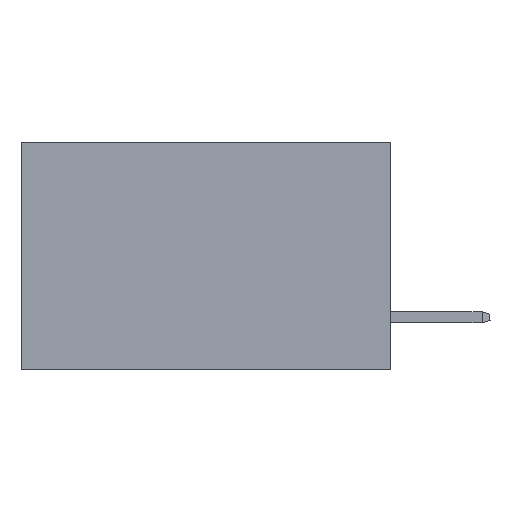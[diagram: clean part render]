
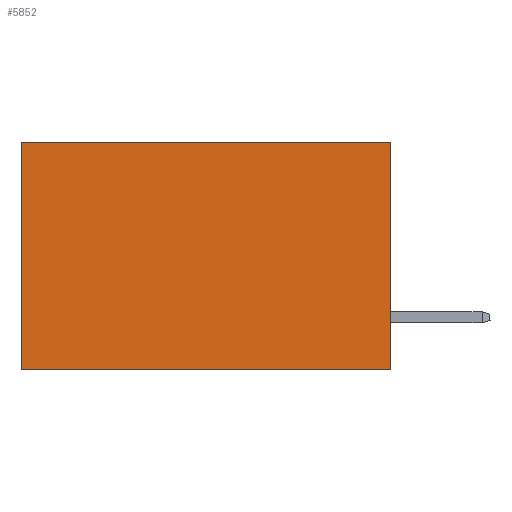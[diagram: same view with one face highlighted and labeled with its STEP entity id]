
A CAD part, left-side view. The second image highlights one B-rep face of the part: STEP entity #5852.
In plain terms, the highlighted planar face has unit normal (-1, 0, 0).
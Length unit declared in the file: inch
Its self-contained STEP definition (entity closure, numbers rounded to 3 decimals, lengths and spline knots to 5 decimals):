
#713 = VERTEX_POINT ( 'NONE', #25586 ) ;
#890 = VERTEX_POINT ( 'NONE', #19324 ) ;
#1612 = EDGE_CURVE ( 'NONE', #20987, #7884, #8159, .T. ) ;
#2070 = VECTOR ( 'NONE', #13593, 39.37008 ) ;
#2595 = EDGE_CURVE ( 'NONE', #890, #713, #14158, .T. ) ;
#3225 = EDGE_CURVE ( 'NONE', #890, #20987, #9853, .T. ) ;
#3799 = VECTOR ( 'NONE', #24616, 39.37008 ) ;
#4770 = EDGE_CURVE ( 'NONE', #713, #7884, #28774, .T. ) ;
#5852 = ADVANCED_FACE ( 'NONE', ( #21918 ), #17741, .F. ) ;
#6243 = DIRECTION ( 'NONE',  ( 1., 0., 0. ) ) ;
#7884 = VERTEX_POINT ( 'NONE', #21443 ) ;
#8159 = LINE ( 'NONE', #26647, #26771 ) ;
#8192 = ORIENTED_EDGE ( 'NONE', *, *, #3225, .T. ) ;
#8851 = CARTESIAN_POINT ( 'NONE',  ( 0.2875, 0., 0. ) ) ;
#8976 = DIRECTION ( 'NONE',  ( 0., 0., -1. ) ) ;
#9764 = DIRECTION ( 'NONE',  ( 0., 1., 0. ) ) ;
#9853 = LINE ( 'NONE', #8851, #3799 ) ;
#10595 = VECTOR ( 'NONE', #9764, 39.37008 ) ;
#11586 = ORIENTED_EDGE ( 'NONE', *, *, #4770, .F. ) ;
#12865 = DIRECTION ( 'NONE',  ( 0., 0., -1. ) ) ;
#13593 = DIRECTION ( 'NONE',  ( 0., 0., -1. ) ) ;
#13962 = CARTESIAN_POINT ( 'NONE',  ( 0.2875, 0., -0.37 ) ) ;
#14158 = LINE ( 'NONE', #17988, #2070 ) ;
#15620 = EDGE_LOOP ( 'NONE', ( #18037, #11586, #22037, #8192 ) ) ;
#17741 = PLANE ( 'NONE',  #24115 ) ;
#17988 = CARTESIAN_POINT ( 'NONE',  ( 0.2875, 0., 0. ) ) ;
#18037 = ORIENTED_EDGE ( 'NONE', *, *, #1612, .T. ) ;
#19324 = CARTESIAN_POINT ( 'NONE',  ( 0.2875, 0., 0. ) ) ;
#20016 = CARTESIAN_POINT ( 'NONE',  ( 0.2875, 0., 0. ) ) ;
#20987 = VERTEX_POINT ( 'NONE', #28680 ) ;
#21443 = CARTESIAN_POINT ( 'NONE',  ( 0.2875, 0.6, -0.37 ) ) ;
#21918 = FACE_OUTER_BOUND ( 'NONE', #15620, .T. ) ;
#22037 = ORIENTED_EDGE ( 'NONE', *, *, #2595, .F. ) ;
#24115 = AXIS2_PLACEMENT_3D ( 'NONE', #20016, #6243, #12865 ) ;
#24616 = DIRECTION ( 'NONE',  ( 0., 1., 0. ) ) ;
#25586 = CARTESIAN_POINT ( 'NONE',  ( 0.2875, 0., -0.37 ) ) ;
#26647 = CARTESIAN_POINT ( 'NONE',  ( 0.2875, 0.6, 0. ) ) ;
#26771 = VECTOR ( 'NONE', #8976, 39.37008 ) ;
#28680 = CARTESIAN_POINT ( 'NONE',  ( 0.2875, 0.6, 0. ) ) ;
#28774 = LINE ( 'NONE', #13962, #10595 ) ;
